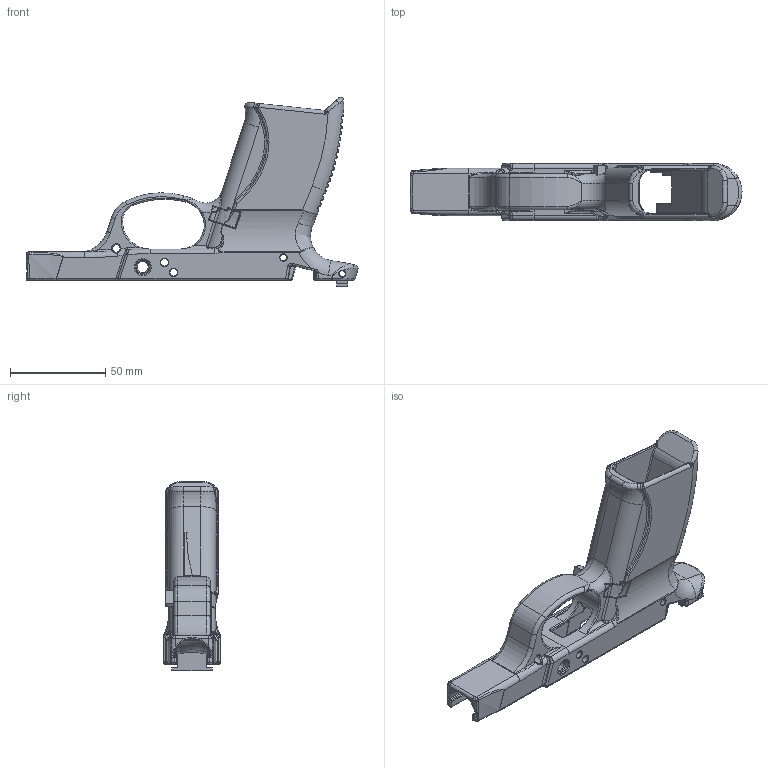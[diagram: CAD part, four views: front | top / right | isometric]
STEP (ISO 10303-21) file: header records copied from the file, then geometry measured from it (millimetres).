
FILE_DESCRIPTION(/* description */ (''),/* implementation_level */ '2;1');
FILE_NAME(/* name */ 'SR9C.step',/* time_stamp */ '2019-11-17T18:05:23-05:00',/* author */ (''),/* organization */ (''),/* preprocessor_version */ 'ST-DEVELOPER v18',/* originating_system */ 'Autodesk Translation Framework v8.12.0.6',/* authorisation */ '');
FILE_SCHEMA (('AUTOMOTIVE_DESIGN { 1 0 10303 214 3 1 1 }'));
Products named in the file (3): SR9C G19 GRIP LENGTH; Mag Catch SR9; SR9 Rear Rail
Assembly tree (2 placements, depth 2):
  SR9C G19 GRIP LENGTH
    Mag Catch SR9
    SR9 Rear Rail
Bounding box: 174.67 x 30 x 99.48 mm (x, y, z)
Volume: 74321.4 mm3; surface area: 44965.9 mm2
Topology: 3 solids, 3 shells, 1490 faces, 3548 edges, 1966 vertices
Faces by surface type: cylinder 518, bspline 498, torus 205, plane 198, sphere 42, cone 29
Full cylindrical faces by diameter (mm): 3.175 x3, 3.5 x1, 4 x6, 4.36 x1, 5.8 x2, 8 x1
Entity records: 57493 total; most frequent: CARTESIAN_POINT 25503, ORIENTED_EDGE 6934, DIRECTION 6374, EDGE_CURVE 3467, AXIS2_PLACEMENT_3D 2644, VERTEX_POINT 1968, EDGE_LOOP 1511, FACE_OUTER_BOUND 1490
